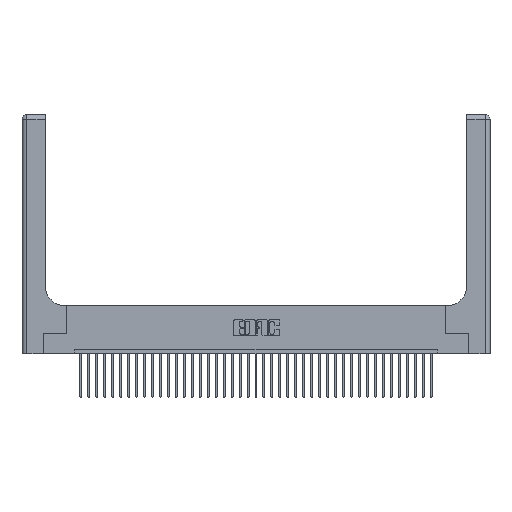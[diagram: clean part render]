
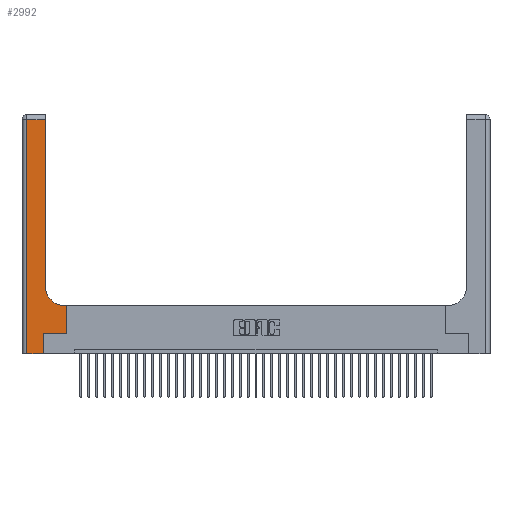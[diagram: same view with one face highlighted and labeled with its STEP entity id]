
A CAD part, top view. The second image highlights one B-rep face of the part: STEP entity #2992.
In plain terms, the highlighted planar face has unit normal (0, 0, 1).
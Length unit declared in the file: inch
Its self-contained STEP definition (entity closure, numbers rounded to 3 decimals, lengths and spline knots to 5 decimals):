
#217 = VERTEX_POINT ( 'NONE', #17421 ) ;
#293 = VECTOR ( 'NONE', #29917, 39.37008 ) ;
#321 = EDGE_LOOP ( 'NONE', ( #37009, #28606, #629, #21506, #6352, #15937, #36389, #35742, #33445 ) ) ;
#607 = CARTESIAN_POINT ( 'NONE',  ( 0.5415, 0.85, 0.37 ) ) ;
#629 = ORIENTED_EDGE ( 'NONE', *, *, #34844, .T. ) ;
#2541 = VECTOR ( 'NONE', #31905, 39.37008 ) ;
#2992 = ADVANCED_FACE ( 'NONE', ( #30808 ), #36056, .F. ) ;
#3204 = CARTESIAN_POINT ( 'NONE',  ( 0., 3., 0.37 ) ) ;
#3681 = DIRECTION ( 'NONE',  ( 1., 0., 0. ) ) ;
#4467 = VECTOR ( 'NONE', #23440, 39.37008 ) ;
#5746 = VERTEX_POINT ( 'NONE', #36356 ) ;
#6352 = ORIENTED_EDGE ( 'NONE', *, *, #22633, .T. ) ;
#6714 = DIRECTION ( 'NONE',  ( 0., 1., 0. ) ) ;
#6743 = LINE ( 'NONE', #33470, #17561 ) ;
#7153 = CARTESIAN_POINT ( 'NONE',  ( 0.5585, 0.25, 0.37 ) ) ;
#7697 = VERTEX_POINT ( 'NONE', #26059 ) ;
#7803 = EDGE_CURVE ( 'NONE', #5746, #217, #30731, .T. ) ;
#8041 = VERTEX_POINT ( 'NONE', #31267 ) ;
#8217 = LINE ( 'NONE', #7153, #34803 ) ;
#8768 = CARTESIAN_POINT ( 'NONE',  ( 0.2915, 0.6, 0.37 ) ) ;
#9531 = LINE ( 'NONE', #37335, #25448 ) ;
#9808 = VERTEX_POINT ( 'NONE', #22477 ) ;
#10299 = CARTESIAN_POINT ( 'NONE',  ( 0.269, 0., 0.37 ) ) ;
#10455 = LINE ( 'NONE', #11372, #2541 ) ;
#11238 = LINE ( 'NONE', #37089, #17871 ) ;
#11372 = CARTESIAN_POINT ( 'NONE',  ( 0.06, 3., 0.37 ) ) ;
#12945 = EDGE_CURVE ( 'NONE', #9808, #7697, #19684, .T. ) ;
#14224 = CARTESIAN_POINT ( 'NONE',  ( 0.5585, 0.25, 0.37 ) ) ;
#14350 = VECTOR ( 'NONE', #31344, 39.37008 ) ;
#14815 = LINE ( 'NONE', #8768, #4467 ) ;
#15937 = ORIENTED_EDGE ( 'NONE', *, *, #32797, .T. ) ;
#16681 = DIRECTION ( 'NONE',  ( 0., 1., 0. ) ) ;
#16927 = CARTESIAN_POINT ( 'NONE',  ( 0.269, 0.25, 0.37 ) ) ;
#17115 = DIRECTION ( 'NONE',  ( 0., 1., 0. ) ) ;
#17225 = EDGE_CURVE ( 'NONE', #7697, #5746, #6743, .T. ) ;
#17421 = CARTESIAN_POINT ( 'NONE',  ( 0.06, 2.94, 0.37 ) ) ;
#17561 = VECTOR ( 'NONE', #6714, 39.37008 ) ;
#17871 = VECTOR ( 'NONE', #16681, 39.37008 ) ;
#18024 = VERTEX_POINT ( 'NONE', #16927 ) ;
#18452 = VERTEX_POINT ( 'NONE', #10299 ) ;
#19684 = CIRCLE ( 'NONE', #36137, 0.25 ) ;
#20838 = EDGE_CURVE ( 'NONE', #8041, #18452, #9531, .T. ) ;
#21234 = DIRECTION ( 'NONE',  ( 0., 0., -1. ) ) ;
#21506 = ORIENTED_EDGE ( 'NONE', *, *, #20838, .T. ) ;
#22477 = CARTESIAN_POINT ( 'NONE',  ( 0.5415, 0.6, 0.37 ) ) ;
#22526 = DIRECTION ( 'NONE',  ( 1., 0., 0. ) ) ;
#22633 = EDGE_CURVE ( 'NONE', #18452, #18024, #11238, .T. ) ;
#23440 = DIRECTION ( 'NONE',  ( -1., 0., 0. ) ) ;
#25297 = EDGE_CURVE ( 'NONE', #29905, #9808, #14815, .T. ) ;
#25448 = VECTOR ( 'NONE', #22526, 39.37008 ) ;
#26059 = CARTESIAN_POINT ( 'NONE',  ( 0.2915, 0.85, 0.37 ) ) ;
#28606 = ORIENTED_EDGE ( 'NONE', *, *, #7803, .T. ) ;
#29321 = LINE ( 'NONE', #32660, #293 ) ;
#29905 = VERTEX_POINT ( 'NONE', #33074 ) ;
#29917 = DIRECTION ( 'NONE',  ( 1., 0., 0. ) ) ;
#30123 = DIRECTION ( 'NONE',  ( -1., 0., 0. ) ) ;
#30415 = VERTEX_POINT ( 'NONE', #14224 ) ;
#30731 = LINE ( 'NONE', #36622, #14350 ) ;
#30808 = FACE_OUTER_BOUND ( 'NONE', #321, .T. ) ;
#31267 = CARTESIAN_POINT ( 'NONE',  ( 0.06, 0., 0.37 ) ) ;
#31344 = DIRECTION ( 'NONE',  ( -1., 0., 0. ) ) ;
#31905 = DIRECTION ( 'NONE',  ( 0., -1., 0. ) ) ;
#32660 = CARTESIAN_POINT ( 'NONE',  ( 0.269, 0.25, 0.37 ) ) ;
#32797 = EDGE_CURVE ( 'NONE', #18024, #30415, #29321, .T. ) ;
#32997 = EDGE_CURVE ( 'NONE', #30415, #29905, #8217, .T. ) ;
#33074 = CARTESIAN_POINT ( 'NONE',  ( 0.5585, 0.6, 0.37 ) ) ;
#33445 = ORIENTED_EDGE ( 'NONE', *, *, #12945, .T. ) ;
#33470 = CARTESIAN_POINT ( 'NONE',  ( 0.2915, 3., 0.37 ) ) ;
#34803 = VECTOR ( 'NONE', #17115, 39.37008 ) ;
#34844 = EDGE_CURVE ( 'NONE', #217, #8041, #10455, .T. ) ;
#35742 = ORIENTED_EDGE ( 'NONE', *, *, #25297, .T. ) ;
#36056 = PLANE ( 'NONE',  #36369 ) ;
#36137 = AXIS2_PLACEMENT_3D ( 'NONE', #607, #36629, #3681 ) ;
#36356 = CARTESIAN_POINT ( 'NONE',  ( 0.2915, 2.94, 0.37 ) ) ;
#36369 = AXIS2_PLACEMENT_3D ( 'NONE', #3204, #21234, #30123 ) ;
#36389 = ORIENTED_EDGE ( 'NONE', *, *, #32997, .T. ) ;
#36622 = CARTESIAN_POINT ( 'NONE',  ( 0., 2.94, 0.37 ) ) ;
#36629 = DIRECTION ( 'NONE',  ( 0., 0., -1. ) ) ;
#37009 = ORIENTED_EDGE ( 'NONE', *, *, #17225, .T. ) ;
#37089 = CARTESIAN_POINT ( 'NONE',  ( 0.269, 0., 0.37 ) ) ;
#37335 = CARTESIAN_POINT ( 'NONE',  ( 0., 0., 0.37 ) ) ;
